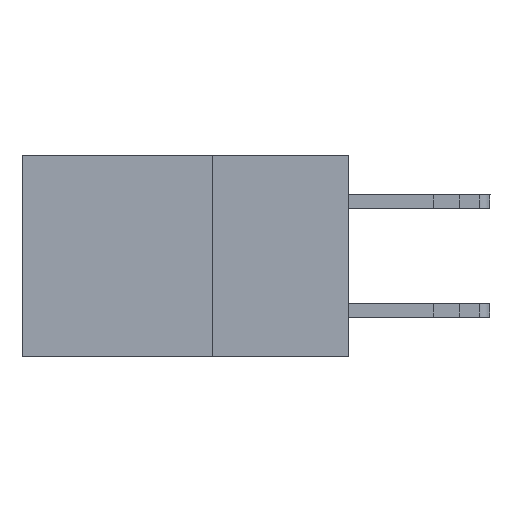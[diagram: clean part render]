
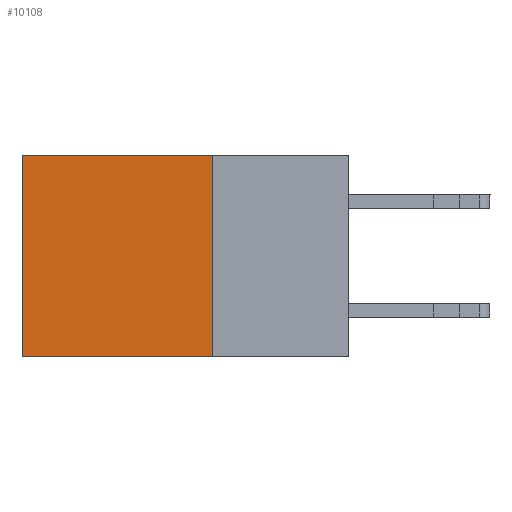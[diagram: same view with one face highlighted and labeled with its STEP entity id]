
A CAD part, left-side view. The second image highlights one B-rep face of the part: STEP entity #10108.
In plain terms, the highlighted planar face has unit normal (-1, 0, 0).
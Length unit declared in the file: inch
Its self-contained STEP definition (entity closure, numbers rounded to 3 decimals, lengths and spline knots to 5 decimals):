
#962 = AXIS2_PLACEMENT_3D ( 'NONE', #3826, #12430, #2948 ) ;
#1611 = ORIENTED_EDGE ( 'NONE', *, *, #4228, .F. ) ;
#2297 = ORIENTED_EDGE ( 'NONE', *, *, #6303, .T. ) ;
#2718 = FACE_OUTER_BOUND ( 'NONE', #3974, .T. ) ;
#2948 = DIRECTION ( 'NONE',  ( 0., 0., -1. ) ) ;
#3165 = VECTOR ( 'NONE', #9011, 39.37008 ) ;
#3591 = CARTESIAN_POINT ( 'NONE',  ( 0.298, 0.25, -0.37 ) ) ;
#3671 = DIRECTION ( 'NONE',  ( 0., 1., 0. ) ) ;
#3826 = CARTESIAN_POINT ( 'NONE',  ( 0.298, 0.25, 0. ) ) ;
#3924 = DIRECTION ( 'NONE',  ( 0., 0., -1. ) ) ;
#3974 = EDGE_LOOP ( 'NONE', ( #2297, #1611, #14710, #10803 ) ) ;
#4063 = VECTOR ( 'NONE', #8805, 39.37008 ) ;
#4228 = EDGE_CURVE ( 'NONE', #9993, #11731, #9591, .T. ) ;
#5129 = VECTOR ( 'NONE', #3924, 39.37008 ) ;
#5450 = LINE ( 'NONE', #13815, #3165 ) ;
#5798 = CARTESIAN_POINT ( 'NONE',  ( 0.298, 0.25, 0. ) ) ;
#6303 = EDGE_CURVE ( 'NONE', #6325, #11731, #5450, .T. ) ;
#6325 = VERTEX_POINT ( 'NONE', #15158 ) ;
#8805 = DIRECTION ( 'NONE',  ( 0., 1., 0. ) ) ;
#8870 = PLANE ( 'NONE',  #962 ) ;
#9011 = DIRECTION ( 'NONE',  ( 0., 0., -1. ) ) ;
#9591 = LINE ( 'NONE', #3591, #14718 ) ;
#9651 = EDGE_CURVE ( 'NONE', #13959, #9993, #14655, .T. ) ;
#9993 = VERTEX_POINT ( 'NONE', #10790 ) ;
#10007 = LINE ( 'NONE', #14800, #4063 ) ;
#10108 = ADVANCED_FACE ( 'NONE', ( #2718 ), #8870, .F. ) ;
#10790 = CARTESIAN_POINT ( 'NONE',  ( 0.298, 0.25, -0.37 ) ) ;
#10803 = ORIENTED_EDGE ( 'NONE', *, *, #15491, .T. ) ;
#11731 = VERTEX_POINT ( 'NONE', #15023 ) ;
#12430 = DIRECTION ( 'NONE',  ( 1., 0., 0. ) ) ;
#12445 = CARTESIAN_POINT ( 'NONE',  ( 0.298, 0.25, 0. ) ) ;
#13815 = CARTESIAN_POINT ( 'NONE',  ( 0.298, 0.6, 0. ) ) ;
#13959 = VERTEX_POINT ( 'NONE', #5798 ) ;
#14655 = LINE ( 'NONE', #12445, #5129 ) ;
#14710 = ORIENTED_EDGE ( 'NONE', *, *, #9651, .F. ) ;
#14718 = VECTOR ( 'NONE', #3671, 39.37008 ) ;
#14800 = CARTESIAN_POINT ( 'NONE',  ( 0.298, 0.25, 0. ) ) ;
#15023 = CARTESIAN_POINT ( 'NONE',  ( 0.298, 0.6, -0.37 ) ) ;
#15158 = CARTESIAN_POINT ( 'NONE',  ( 0.298, 0.6, 0. ) ) ;
#15491 = EDGE_CURVE ( 'NONE', #13959, #6325, #10007, .T. ) ;
